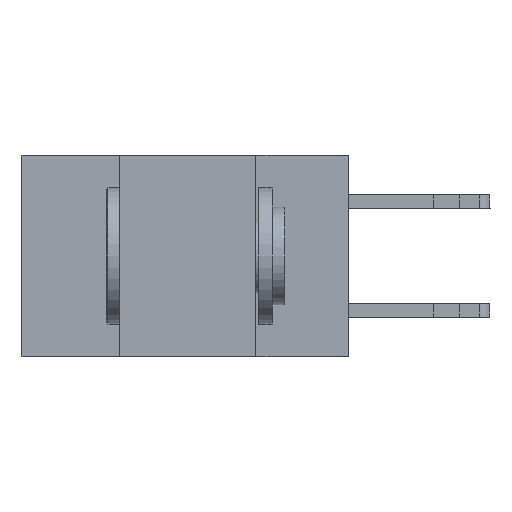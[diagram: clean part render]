
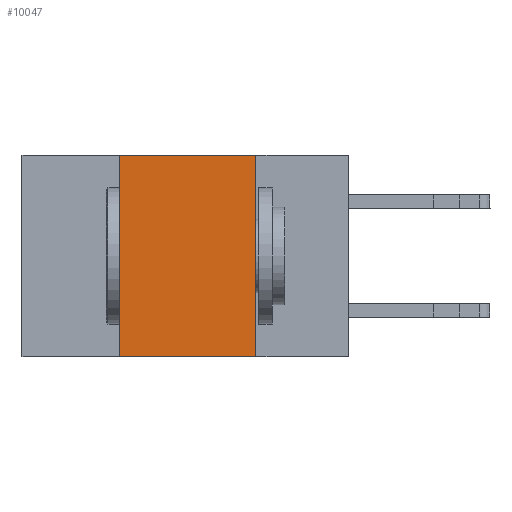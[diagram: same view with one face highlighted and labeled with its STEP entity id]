
A CAD part, left-side view. The second image highlights one B-rep face of the part: STEP entity #10047.
In plain terms, the highlighted planar face has unit normal (-1, 0, 0).
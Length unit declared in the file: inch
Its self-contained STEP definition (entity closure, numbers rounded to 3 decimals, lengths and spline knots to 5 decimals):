
#68 = CARTESIAN_POINT ( 'NONE',  ( 0., 0.17, -0.37 ) ) ;
#221 = CARTESIAN_POINT ( 'NONE',  ( 0., 0.6, 0. ) ) ;
#318 = DIRECTION ( 'NONE',  ( 0., 0., -1. ) ) ;
#779 = CARTESIAN_POINT ( 'NONE',  ( 0., 0.42, -0.37 ) ) ;
#1678 = VECTOR ( 'NONE', #4937, 39.37008 ) ;
#1943 = LINE ( 'NONE', #7034, #10087 ) ;
#1957 = DIRECTION ( 'NONE',  ( 0., -1., 0. ) ) ;
#2063 = CARTESIAN_POINT ( 'NONE',  ( 0., 0.6, -0.37 ) ) ;
#2893 = CARTESIAN_POINT ( 'NONE',  ( 0., 0.6, 0. ) ) ;
#2978 = CARTESIAN_POINT ( 'NONE',  ( 0., 0.17, -0.37 ) ) ;
#3813 = PLANE ( 'NONE',  #9904 ) ;
#3869 = FACE_OUTER_BOUND ( 'NONE', #5568, .T. ) ;
#4816 = ORIENTED_EDGE ( 'NONE', *, *, #6021, .F. ) ;
#4937 = DIRECTION ( 'NONE',  ( 0., 0., -1. ) ) ;
#5568 = EDGE_LOOP ( 'NONE', ( #9051, #4816, #9427, #5958 ) ) ;
#5958 = ORIENTED_EDGE ( 'NONE', *, *, #9070, .T. ) ;
#5973 = VERTEX_POINT ( 'NONE', #9833 ) ;
#6021 = EDGE_CURVE ( 'NONE', #5973, #10256, #8064, .T. ) ;
#6545 = VECTOR ( 'NONE', #7209, 39.37008 ) ;
#6802 = VERTEX_POINT ( 'NONE', #779 ) ;
#7034 = CARTESIAN_POINT ( 'NONE',  ( 0., 0.42, -0.37 ) ) ;
#7209 = DIRECTION ( 'NONE',  ( 0., -1., 0. ) ) ;
#7724 = VERTEX_POINT ( 'NONE', #68 ) ;
#8064 = LINE ( 'NONE', #221, #6545 ) ;
#8863 = DIRECTION ( 'NONE',  ( 0., 0., 1. ) ) ;
#9051 = ORIENTED_EDGE ( 'NONE', *, *, #9247, .F. ) ;
#9070 = EDGE_CURVE ( 'NONE', #6802, #7724, #9794, .T. ) ;
#9247 = EDGE_CURVE ( 'NONE', #10256, #7724, #9963, .T. ) ;
#9427 = ORIENTED_EDGE ( 'NONE', *, *, #9503, .F. ) ;
#9503 = EDGE_CURVE ( 'NONE', #6802, #5973, #1943, .T. ) ;
#9794 = LINE ( 'NONE', #2063, #11003 ) ;
#9833 = CARTESIAN_POINT ( 'NONE',  ( 0., 0.42, 0. ) ) ;
#9904 = AXIS2_PLACEMENT_3D ( 'NONE', #2893, #10849, #318 ) ;
#9963 = LINE ( 'NONE', #2978, #1678 ) ;
#10047 = ADVANCED_FACE ( 'NONE', ( #3869 ), #3813, .F. ) ;
#10087 = VECTOR ( 'NONE', #8863, 39.37008 ) ;
#10211 = CARTESIAN_POINT ( 'NONE',  ( 0., 0.17, 0. ) ) ;
#10256 = VERTEX_POINT ( 'NONE', #10211 ) ;
#10849 = DIRECTION ( 'NONE',  ( 1., 0., 0. ) ) ;
#11003 = VECTOR ( 'NONE', #1957, 39.37008 ) ;
